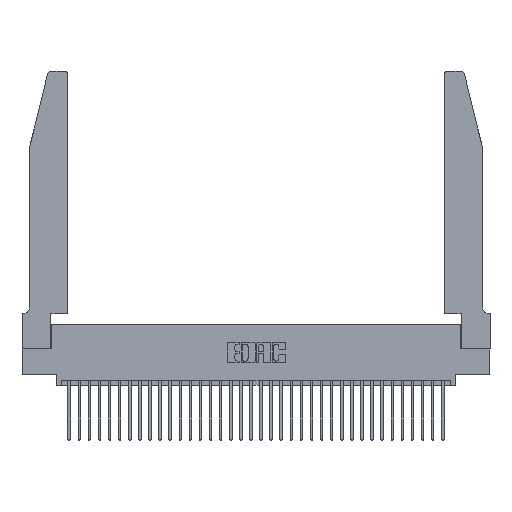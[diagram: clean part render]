
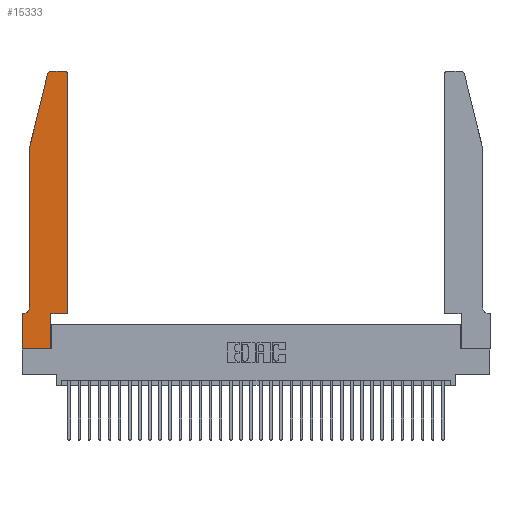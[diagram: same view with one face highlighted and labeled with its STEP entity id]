
A CAD part, top view. The second image highlights one B-rep face of the part: STEP entity #15333.
In plain terms, the highlighted planar face has unit normal (0, 0, 1).
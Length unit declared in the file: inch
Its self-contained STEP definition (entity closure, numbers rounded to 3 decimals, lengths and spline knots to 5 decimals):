
#293 = DIRECTION ( 'NONE',  ( 0., 0., -1. ) ) ;
#397 = CARTESIAN_POINT ( 'NONE',  ( 0., 0.35, 0.37 ) ) ;
#608 = DIRECTION ( 'NONE',  ( 1., 0., 0. ) ) ;
#1123 = CARTESIAN_POINT ( 'NONE',  ( 0.4505, 0.35, 0.37 ) ) ;
#1166 = ORIENTED_EDGE ( 'NONE', *, *, #24536, .T. ) ;
#1821 = VERTEX_POINT ( 'NONE', #8179 ) ;
#2086 = DIRECTION ( 'NONE',  ( 0., 0., 1. ) ) ;
#2363 = LINE ( 'NONE', #1123, #16111 ) ;
#2853 = CARTESIAN_POINT ( 'NONE',  ( 0.0755, 2., 0.37 ) ) ;
#3583 = VECTOR ( 'NONE', #23095, 39.37008 ) ;
#3854 = ORIENTED_EDGE ( 'NONE', *, *, #28966, .T. ) ;
#4121 = FACE_OUTER_BOUND ( 'NONE', #26809, .T. ) ;
#4251 = VERTEX_POINT ( 'NONE', #34076 ) ;
#4422 = VERTEX_POINT ( 'NONE', #34751 ) ;
#5457 = AXIS2_PLACEMENT_3D ( 'NONE', #16730, #293, #19465 ) ;
#5623 = CARTESIAN_POINT ( 'NONE',  ( 0.0755, 0.35, 0.37 ) ) ;
#5741 = DIRECTION ( 'NONE',  ( -1., 0., 0. ) ) ;
#5870 = DIRECTION ( 'NONE',  ( 1., 0., 0. ) ) ;
#6026 = ORIENTED_EDGE ( 'NONE', *, *, #27366, .T. ) ;
#6225 = ORIENTED_EDGE ( 'NONE', *, *, #10713, .T. ) ;
#6260 = VERTEX_POINT ( 'NONE', #27402 ) ;
#6402 = CARTESIAN_POINT ( 'NONE',  ( 0.2865, 0.35, 0.37 ) ) ;
#6663 = LINE ( 'NONE', #22444, #33876 ) ;
#6703 = CIRCLE ( 'NONE', #9979, 0.03 ) ;
#6875 = EDGE_CURVE ( 'NONE', #27052, #30153, #9278, .T. ) ;
#7111 = ORIENTED_EDGE ( 'NONE', *, *, #18871, .T. ) ;
#7805 = EDGE_CURVE ( 'NONE', #21199, #25791, #2363, .T. ) ;
#7906 = ORIENTED_EDGE ( 'NONE', *, *, #26024, .T. ) ;
#8032 = CIRCLE ( 'NONE', #5457, 0.07 ) ;
#8179 = CARTESIAN_POINT ( 'NONE',  ( 0.4205, 2.75, 0.37 ) ) ;
#9278 = LINE ( 'NONE', #5623, #29297 ) ;
#9979 = AXIS2_PLACEMENT_3D ( 'NONE', #33257, #17044, #608 ) ;
#10713 = EDGE_CURVE ( 'NONE', #6260, #21199, #22287, .T. ) ;
#10762 = EDGE_CURVE ( 'NONE', #30594, #6260, #34124, .T. ) ;
#11396 = CARTESIAN_POINT ( 'NONE',  ( 0., 0., 0.37 ) ) ;
#13201 = VERTEX_POINT ( 'NONE', #2853 ) ;
#13902 = EDGE_CURVE ( 'NONE', #19370, #27052, #8032, .T. ) ;
#14179 = CARTESIAN_POINT ( 'NONE',  ( 0.4505, 0.35, 0.37 ) ) ;
#14195 = VECTOR ( 'NONE', #33398, 39.37008 ) ;
#14430 = CARTESIAN_POINT ( 'NONE',  ( 0.4505, 0.35, 0.37 ) ) ;
#14607 = DIRECTION ( 'NONE',  ( 0., 0., 1. ) ) ;
#14628 = CARTESIAN_POINT ( 'NONE',  ( 0.0755, 0.42, 0.37 ) ) ;
#14894 = ORIENTED_EDGE ( 'NONE', *, *, #7805, .T. ) ;
#15046 = EDGE_CURVE ( 'NONE', #1821, #30264, #6663, .T. ) ;
#15333 = ADVANCED_FACE ( 'NONE', ( #4121 ), #18532, .T. ) ;
#16111 = VECTOR ( 'NONE', #23001, 39.37008 ) ;
#16479 = ORIENTED_EDGE ( 'NONE', *, *, #10762, .T. ) ;
#16730 = CARTESIAN_POINT ( 'NONE',  ( 0.0055, 0.42, 0.37 ) ) ;
#17044 = DIRECTION ( 'NONE',  ( 0., 0., 1. ) ) ;
#17714 = EDGE_CURVE ( 'NONE', #13201, #19370, #30796, .T. ) ;
#18420 = CARTESIAN_POINT ( 'NONE',  ( 0., 0.35, 0.37 ) ) ;
#18489 = CARTESIAN_POINT ( 'NONE',  ( 0.0055, 0.35, 0.37 ) ) ;
#18532 = PLANE ( 'NONE',  #21071 ) ;
#18871 = EDGE_CURVE ( 'NONE', #4422, #13201, #32534, .T. ) ;
#19370 = VERTEX_POINT ( 'NONE', #14628 ) ;
#19465 = DIRECTION ( 'NONE',  ( -1., 0., 0. ) ) ;
#21037 = CARTESIAN_POINT ( 'NONE',  ( 0.0755, 2., 0.37 ) ) ;
#21071 = AXIS2_PLACEMENT_3D ( 'NONE', #18420, #2086, #21250 ) ;
#21199 = VERTEX_POINT ( 'NONE', #14179 ) ;
#21250 = DIRECTION ( 'NONE',  ( 1., 0., 0. ) ) ;
#21312 = CARTESIAN_POINT ( 'NONE',  ( 0.2865, 0., 0.37 ) ) ;
#21430 = LINE ( 'NONE', #27185, #34950 ) ;
#21540 = ORIENTED_EDGE ( 'NONE', *, *, #13902, .T. ) ;
#21703 = ORIENTED_EDGE ( 'NONE', *, *, #15046, .T. ) ;
#21839 = ORIENTED_EDGE ( 'NONE', *, *, #6875, .T. ) ;
#22287 = LINE ( 'NONE', #14430, #14195 ) ;
#22444 = CARTESIAN_POINT ( 'NONE',  ( 0.2605, 2.75, 0.37 ) ) ;
#22855 = DIRECTION ( 'NONE',  ( 0., 1., 0. ) ) ;
#23001 = DIRECTION ( 'NONE',  ( 0., 1., 0. ) ) ;
#23095 = DIRECTION ( 'NONE',  ( -0.239, -0.971, 0. ) ) ;
#24066 = ORIENTED_EDGE ( 'NONE', *, *, #17714, .T. ) ;
#24441 = VECTOR ( 'NONE', #31791, 39.37008 ) ;
#24536 = EDGE_CURVE ( 'NONE', #30153, #4251, #21430, .T. ) ;
#25203 = DIRECTION ( 'NONE',  ( -1., 0., 0. ) ) ;
#25223 = CARTESIAN_POINT ( 'NONE',  ( 0.4505, 2.72, 0.37 ) ) ;
#25791 = VERTEX_POINT ( 'NONE', #25223 ) ;
#26024 = EDGE_CURVE ( 'NONE', #30264, #4422, #26865, .T. ) ;
#26699 = VECTOR ( 'NONE', #5870, 39.37008 ) ;
#26809 = EDGE_LOOP ( 'NONE', ( #21703, #7906, #7111, #24066, #21540, #21839, #1166, #3854, #16479, #6225, #14894, #6026 ) ) ;
#26865 = CIRCLE ( 'NONE', #27312, 0.03 ) ;
#27052 = VERTEX_POINT ( 'NONE', #18489 ) ;
#27185 = CARTESIAN_POINT ( 'NONE',  ( 0., 0., 0.37 ) ) ;
#27312 = AXIS2_PLACEMENT_3D ( 'NONE', #30875, #14607, #33570 ) ;
#27366 = EDGE_CURVE ( 'NONE', #25791, #1821, #6703, .T. ) ;
#27402 = CARTESIAN_POINT ( 'NONE',  ( 0.2865, 0.35, 0.37 ) ) ;
#28966 = EDGE_CURVE ( 'NONE', #4251, #30594, #29251, .T. ) ;
#29251 = LINE ( 'NONE', #11396, #26699 ) ;
#29297 = VECTOR ( 'NONE', #5741, 39.37008 ) ;
#29903 = DIRECTION ( 'NONE',  ( 0., -1., 0. ) ) ;
#30153 = VERTEX_POINT ( 'NONE', #397 ) ;
#30264 = VERTEX_POINT ( 'NONE', #33510 ) ;
#30594 = VERTEX_POINT ( 'NONE', #21312 ) ;
#30796 = LINE ( 'NONE', #21037, #24441 ) ;
#30875 = CARTESIAN_POINT ( 'NONE',  ( 0.284, 2.72, 0.37 ) ) ;
#31791 = DIRECTION ( 'NONE',  ( 0., -1., 0. ) ) ;
#32534 = LINE ( 'NONE', #33849, #3583 ) ;
#33257 = CARTESIAN_POINT ( 'NONE',  ( 0.4205, 2.72, 0.37 ) ) ;
#33279 = VECTOR ( 'NONE', #22855, 39.37008 ) ;
#33398 = DIRECTION ( 'NONE',  ( 1., 0., 0. ) ) ;
#33510 = CARTESIAN_POINT ( 'NONE',  ( 0.284, 2.75, 0.37 ) ) ;
#33570 = DIRECTION ( 'NONE',  ( 1., 0., 0. ) ) ;
#33849 = CARTESIAN_POINT ( 'NONE',  ( 0.0755, 2., 0.37 ) ) ;
#33876 = VECTOR ( 'NONE', #25203, 39.37008 ) ;
#34076 = CARTESIAN_POINT ( 'NONE',  ( 0., 0., 0.37 ) ) ;
#34124 = LINE ( 'NONE', #6402, #33279 ) ;
#34751 = CARTESIAN_POINT ( 'NONE',  ( 0.25487, 2.72718, 0.37 ) ) ;
#34950 = VECTOR ( 'NONE', #29903, 39.37008 ) ;
